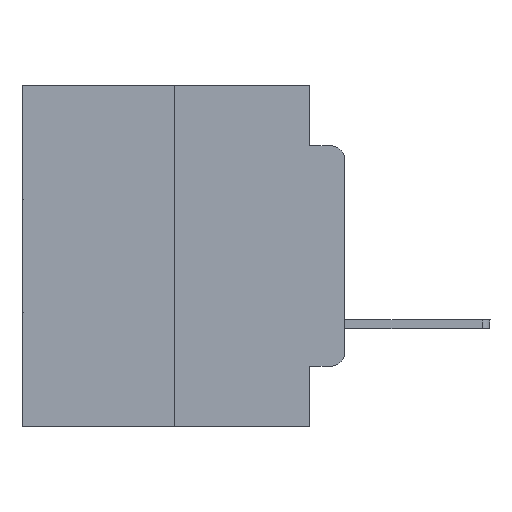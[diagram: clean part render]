
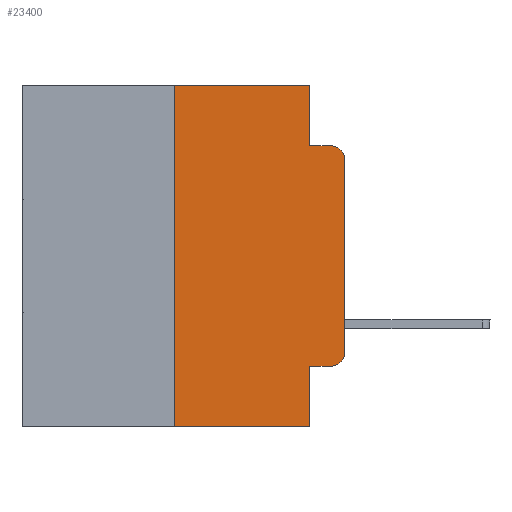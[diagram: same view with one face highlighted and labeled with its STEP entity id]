
A CAD part, left-side view. The second image highlights one B-rep face of the part: STEP entity #23400.
In plain terms, the highlighted planar face has unit normal (-1, 0, 0).
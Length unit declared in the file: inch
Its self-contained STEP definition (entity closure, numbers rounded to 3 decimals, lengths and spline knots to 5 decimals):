
#877 = AXIS2_PLACEMENT_3D ( 'NONE', #3950, #20314, #7898 ) ;
#1042 = CARTESIAN_POINT ( 'NONE',  ( 0., 0.473, 0. ) ) ;
#1392 = DIRECTION ( 'NONE',  ( 0., 0., -1. ) ) ;
#1415 = ORIENTED_EDGE ( 'NONE', *, *, #16562, .F. ) ;
#2022 = DIRECTION ( 'NONE',  ( 0., 0., -1. ) ) ;
#2218 = VECTOR ( 'NONE', #4256, 39.37008 ) ;
#2789 = ORIENTED_EDGE ( 'NONE', *, *, #17117, .T. ) ;
#2935 = VERTEX_POINT ( 'NONE', #21140 ) ;
#3159 = CIRCLE ( 'NONE', #877, 0.02 ) ;
#3265 = VECTOR ( 'NONE', #2022, 39.37008 ) ;
#3516 = DIRECTION ( 'NONE',  ( 0., 0., 1. ) ) ;
#3925 = VERTEX_POINT ( 'NONE', #23224 ) ;
#3950 = CARTESIAN_POINT ( 'NONE',  ( 0., 0.02, -0.1085 ) ) ;
#4251 = EDGE_CURVE ( 'NONE', #2935, #9081, #11127, .T. ) ;
#4256 = DIRECTION ( 'NONE',  ( 0., -1., 0. ) ) ;
#4690 = DIRECTION ( 'NONE',  ( -1., 0., 0. ) ) ;
#4702 = VERTEX_POINT ( 'NONE', #21732 ) ;
#5248 = ORIENTED_EDGE ( 'NONE', *, *, #12740, .T. ) ;
#5459 = CARTESIAN_POINT ( 'NONE',  ( 0., 0.051, 0. ) ) ;
#7362 = ORIENTED_EDGE ( 'NONE', *, *, #4251, .F. ) ;
#7564 = VERTEX_POINT ( 'NONE', #18661 ) ;
#7898 = DIRECTION ( 'NONE',  ( 0., 0., -1. ) ) ;
#7901 = CARTESIAN_POINT ( 'NONE',  ( 0., 0.051, 0. ) ) ;
#8557 = EDGE_CURVE ( 'NONE', #10460, #4702, #25741, .T. ) ;
#8691 = VECTOR ( 'NONE', #17150, 39.37008 ) ;
#9081 = VERTEX_POINT ( 'NONE', #20091 ) ;
#9792 = VERTEX_POINT ( 'NONE', #20797 ) ;
#10114 = CARTESIAN_POINT ( 'NONE',  ( 0., 0.473, 0. ) ) ;
#10126 = ORIENTED_EDGE ( 'NONE', *, *, #15456, .F. ) ;
#10318 = CARTESIAN_POINT ( 'NONE',  ( 0., 0.051, -0.5 ) ) ;
#10460 = VERTEX_POINT ( 'NONE', #12624 ) ;
#10982 = ORIENTED_EDGE ( 'NONE', *, *, #11427, .F. ) ;
#11127 = LINE ( 'NONE', #22296, #18609 ) ;
#11142 = VERTEX_POINT ( 'NONE', #7901 ) ;
#11427 = EDGE_CURVE ( 'NONE', #11142, #9792, #25745, .T. ) ;
#12025 = VERTEX_POINT ( 'NONE', #26079 ) ;
#12433 = CARTESIAN_POINT ( 'NONE',  ( 0., 0.051, -0.0885 ) ) ;
#12530 = CARTESIAN_POINT ( 'NONE',  ( 0., 0.051, 0. ) ) ;
#12624 = CARTESIAN_POINT ( 'NONE',  ( 0., 0.02, -0.4115 ) ) ;
#12740 = EDGE_CURVE ( 'NONE', #12025, #10460, #15029, .T. ) ;
#13369 = DIRECTION ( 'NONE',  ( 0., 0., 1. ) ) ;
#13426 = EDGE_LOOP ( 'NONE', ( #18237, #2789, #19267, #10982, #1415, #7362, #15658, #10126, #5248, #26589 ) ) ;
#14115 = EDGE_CURVE ( 'NONE', #9792, #3925, #25231, .T. ) ;
#14997 = CARTESIAN_POINT ( 'NONE',  ( 0., 0.02, -0.3915 ) ) ;
#15029 = LINE ( 'NONE', #25695, #20833 ) ;
#15168 = CARTESIAN_POINT ( 'NONE',  ( 0., 0., 0. ) ) ;
#15251 = DIRECTION ( 'NONE',  ( 0., 0., -1. ) ) ;
#15265 = PLANE ( 'NONE',  #20243 ) ;
#15442 = DIRECTION ( 'NONE',  ( 0., 0., -1. ) ) ;
#15456 = EDGE_CURVE ( 'NONE', #12025, #21148, #21995, .T. ) ;
#15658 = ORIENTED_EDGE ( 'NONE', *, *, #21460, .T. ) ;
#15842 = LINE ( 'NONE', #21045, #8691 ) ;
#16562 = EDGE_CURVE ( 'NONE', #9081, #11142, #21621, .T. ) ;
#17004 = VECTOR ( 'NONE', #1392, 39.37008 ) ;
#17117 = EDGE_CURVE ( 'NONE', #7564, #3925, #3159, .T. ) ;
#17150 = DIRECTION ( 'NONE',  ( 0., -1., 0. ) ) ;
#18237 = ORIENTED_EDGE ( 'NONE', *, *, #20172, .T. ) ;
#18609 = VECTOR ( 'NONE', #3516, 39.37008 ) ;
#18661 = CARTESIAN_POINT ( 'NONE',  ( 0., 0., -0.1085 ) ) ;
#18998 = DIRECTION ( 'NONE',  ( 0., -1., 0. ) ) ;
#19267 = ORIENTED_EDGE ( 'NONE', *, *, #14115, .F. ) ;
#19411 = DIRECTION ( 'NONE',  ( 1., 0., 0. ) ) ;
#19549 = DIRECTION ( 'NONE',  ( 0., -1., 0. ) ) ;
#20091 = CARTESIAN_POINT ( 'NONE',  ( 0., 0.25, 0. ) ) ;
#20172 = EDGE_CURVE ( 'NONE', #4702, #7564, #22367, .T. ) ;
#20243 = AXIS2_PLACEMENT_3D ( 'NONE', #1042, #19411, #15442 ) ;
#20314 = DIRECTION ( 'NONE',  ( -1., 0., 0. ) ) ;
#20631 = FACE_OUTER_BOUND ( 'NONE', #13426, .T. ) ;
#20797 = CARTESIAN_POINT ( 'NONE',  ( 0., 0.051, -0.0885 ) ) ;
#20833 = VECTOR ( 'NONE', #19549, 39.37008 ) ;
#21023 = AXIS2_PLACEMENT_3D ( 'NONE', #14997, #4690, #15251 ) ;
#21045 = CARTESIAN_POINT ( 'NONE',  ( 0., 0.473, -0.5 ) ) ;
#21140 = CARTESIAN_POINT ( 'NONE',  ( 0., 0.25, -0.5 ) ) ;
#21148 = VERTEX_POINT ( 'NONE', #10318 ) ;
#21421 = VECTOR ( 'NONE', #13369, 39.37008 ) ;
#21460 = EDGE_CURVE ( 'NONE', #2935, #21148, #15842, .T. ) ;
#21621 = LINE ( 'NONE', #10114, #2218 ) ;
#21732 = CARTESIAN_POINT ( 'NONE',  ( 0., 0., -0.3915 ) ) ;
#21995 = LINE ( 'NONE', #12530, #3265 ) ;
#22296 = CARTESIAN_POINT ( 'NONE',  ( 0., 0.25, 0. ) ) ;
#22367 = LINE ( 'NONE', #15168, #21421 ) ;
#23224 = CARTESIAN_POINT ( 'NONE',  ( 0., 0.02, -0.0885 ) ) ;
#23400 = ADVANCED_FACE ( 'NONE', ( #20631 ), #15265, .F. ) ;
#23623 = VECTOR ( 'NONE', #18998, 39.37008 ) ;
#25231 = LINE ( 'NONE', #12433, #23623 ) ;
#25695 = CARTESIAN_POINT ( 'NONE',  ( 0., 0.051, -0.4115 ) ) ;
#25741 = CIRCLE ( 'NONE', #21023, 0.02 ) ;
#25745 = LINE ( 'NONE', #5459, #17004 ) ;
#26079 = CARTESIAN_POINT ( 'NONE',  ( 0., 0.051, -0.4115 ) ) ;
#26589 = ORIENTED_EDGE ( 'NONE', *, *, #8557, .T. ) ;
